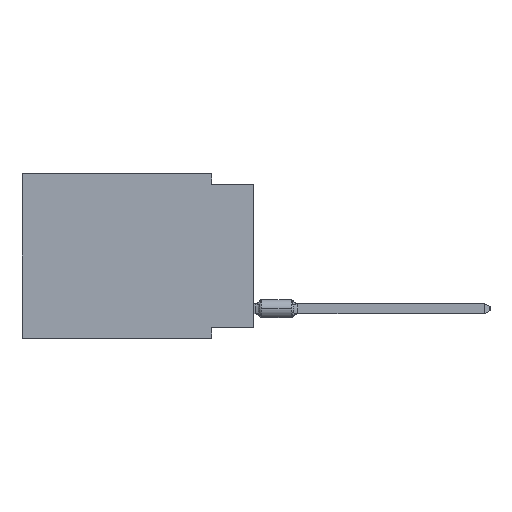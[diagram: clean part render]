
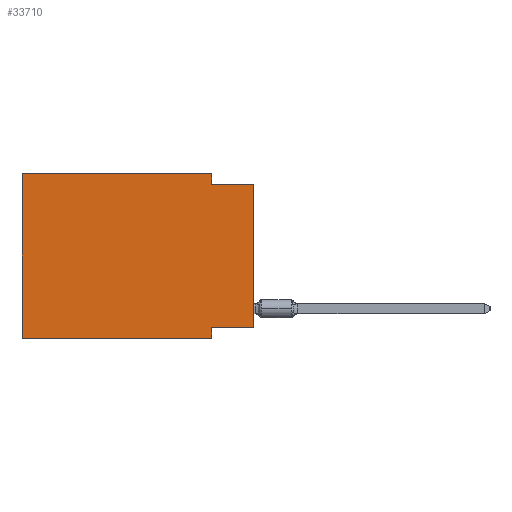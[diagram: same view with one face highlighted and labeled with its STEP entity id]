
A CAD part, left-side view. The second image highlights one B-rep face of the part: STEP entity #33710.
In plain terms, the highlighted planar face has unit normal (-1, 0, 0).
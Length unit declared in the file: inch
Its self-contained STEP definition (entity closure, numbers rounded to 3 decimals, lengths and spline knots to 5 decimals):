
#37 = ORIENTED_EDGE ( 'NONE', *, *, #62863, .F. ) ;
#755 = EDGE_CURVE ( 'NONE', #65345, #5390, #43578, .T. ) ;
#1181 = CARTESIAN_POINT ( 'NONE',  ( 0., 0.55, 0. ) ) ;
#2439 = DIRECTION ( 'NONE',  ( 0., -1., 0. ) ) ;
#3043 = CARTESIAN_POINT ( 'NONE',  ( 0., 0., -0.025 ) ) ;
#4027 = EDGE_CURVE ( 'NONE', #24938, #4517, #44530, .T. ) ;
#4517 = VERTEX_POINT ( 'NONE', #8158 ) ;
#5390 = VERTEX_POINT ( 'NONE', #9267 ) ;
#5604 = VERTEX_POINT ( 'NONE', #17944 ) ;
#6189 = CARTESIAN_POINT ( 'NONE',  ( 0., 0.1, 0. ) ) ;
#6747 = PLANE ( 'NONE',  #20320 ) ;
#8158 = CARTESIAN_POINT ( 'NONE',  ( 0., 0., -0.025 ) ) ;
#8876 = VECTOR ( 'NONE', #11749, 39.37008 ) ;
#8984 = VECTOR ( 'NONE', #13253, 39.37008 ) ;
#9267 = CARTESIAN_POINT ( 'NONE',  ( 0., 0.1, -0.39 ) ) ;
#11488 = CARTESIAN_POINT ( 'NONE',  ( 0., 0.1, -0.39 ) ) ;
#11749 = DIRECTION ( 'NONE',  ( 0., 0., -1. ) ) ;
#11923 = CARTESIAN_POINT ( 'NONE',  ( 0., 0.55, 0. ) ) ;
#12155 = VECTOR ( 'NONE', #2439, 39.37008 ) ;
#13039 = EDGE_CURVE ( 'NONE', #24938, #65345, #42790, .T. ) ;
#13166 = LINE ( 'NONE', #3043, #29768 ) ;
#13253 = DIRECTION ( 'NONE',  ( 0., -1., 0. ) ) ;
#13593 = EDGE_LOOP ( 'NONE', ( #61643, #64177, #41703, #37, #20836, #57569, #29453, #67343 ) ) ;
#15653 = EDGE_CURVE ( 'NONE', #36154, #5390, #22679, .T. ) ;
#16733 = DIRECTION ( 'NONE',  ( 0., 0., -1. ) ) ;
#17944 = CARTESIAN_POINT ( 'NONE',  ( 0., 0.1, -0.025 ) ) ;
#20320 = AXIS2_PLACEMENT_3D ( 'NONE', #22767, #44056, #39174 ) ;
#20350 = EDGE_CURVE ( 'NONE', #5604, #4517, #13166, .T. ) ;
#20721 = VECTOR ( 'NONE', #16733, 39.37008 ) ;
#20836 = ORIENTED_EDGE ( 'NONE', *, *, #50996, .F. ) ;
#22679 = LINE ( 'NONE', #39087, #8984 ) ;
#22767 = CARTESIAN_POINT ( 'NONE',  ( 0., 0.55, 0. ) ) ;
#22944 = CARTESIAN_POINT ( 'NONE',  ( 0., 0.1, -0.365 ) ) ;
#24938 = VERTEX_POINT ( 'NONE', #26379 ) ;
#26379 = CARTESIAN_POINT ( 'NONE',  ( 0., 0., -0.365 ) ) ;
#26388 = DIRECTION ( 'NONE',  ( 0., 1., 0. ) ) ;
#29453 = ORIENTED_EDGE ( 'NONE', *, *, #755, .F. ) ;
#29768 = VECTOR ( 'NONE', #34791, 39.37008 ) ;
#33710 = ADVANCED_FACE ( 'NONE', ( #59069 ), #6747, .F. ) ;
#33716 = CARTESIAN_POINT ( 'NONE',  ( 0., 0., 0. ) ) ;
#34791 = DIRECTION ( 'NONE',  ( 0., -1., 0. ) ) ;
#36154 = VERTEX_POINT ( 'NONE', #36719 ) ;
#36719 = CARTESIAN_POINT ( 'NONE',  ( 0., 0.55, -0.39 ) ) ;
#37216 = CARTESIAN_POINT ( 'NONE',  ( 0., 0., -0.365 ) ) ;
#39087 = CARTESIAN_POINT ( 'NONE',  ( 0., 0.55, -0.39 ) ) ;
#39174 = DIRECTION ( 'NONE',  ( 0., 0., -1. ) ) ;
#41703 = ORIENTED_EDGE ( 'NONE', *, *, #44274, .F. ) ;
#42790 = LINE ( 'NONE', #37216, #45687 ) ;
#43578 = LINE ( 'NONE', #11488, #20721 ) ;
#44056 = DIRECTION ( 'NONE',  ( 1., 0., 0. ) ) ;
#44274 = EDGE_CURVE ( 'NONE', #60000, #5604, #57220, .T. ) ;
#44530 = LINE ( 'NONE', #33716, #52191 ) ;
#45687 = VECTOR ( 'NONE', #26388, 39.37008 ) ;
#50996 = EDGE_CURVE ( 'NONE', #36154, #55534, #67262, .T. ) ;
#52191 = VECTOR ( 'NONE', #65113, 39.37008 ) ;
#55534 = VERTEX_POINT ( 'NONE', #1181 ) ;
#57220 = LINE ( 'NONE', #6189, #8876 ) ;
#57569 = ORIENTED_EDGE ( 'NONE', *, *, #15653, .T. ) ;
#59069 = FACE_OUTER_BOUND ( 'NONE', #13593, .T. ) ;
#60000 = VERTEX_POINT ( 'NONE', #64053 ) ;
#61643 = ORIENTED_EDGE ( 'NONE', *, *, #4027, .T. ) ;
#61678 = VECTOR ( 'NONE', #65628, 39.37008 ) ;
#62863 = EDGE_CURVE ( 'NONE', #55534, #60000, #66266, .T. ) ;
#64053 = CARTESIAN_POINT ( 'NONE',  ( 0., 0.1, 0. ) ) ;
#64177 = ORIENTED_EDGE ( 'NONE', *, *, #20350, .F. ) ;
#65113 = DIRECTION ( 'NONE',  ( 0., 0., 1. ) ) ;
#65345 = VERTEX_POINT ( 'NONE', #22944 ) ;
#65628 = DIRECTION ( 'NONE',  ( 0., 0., 1. ) ) ;
#65922 = CARTESIAN_POINT ( 'NONE',  ( 0., 0.55, 0. ) ) ;
#66266 = LINE ( 'NONE', #65922, #12155 ) ;
#67262 = LINE ( 'NONE', #11923, #61678 ) ;
#67343 = ORIENTED_EDGE ( 'NONE', *, *, #13039, .F. ) ;
